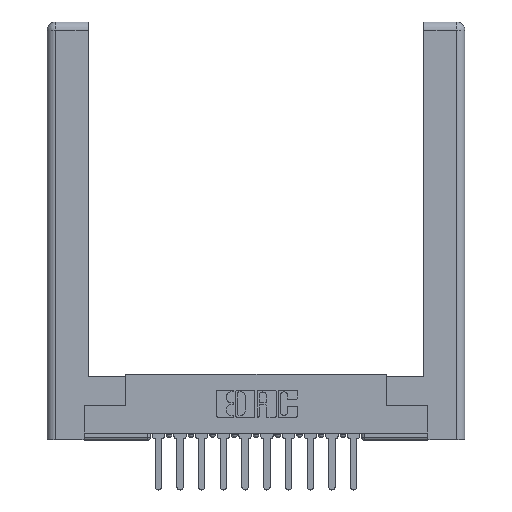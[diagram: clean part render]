
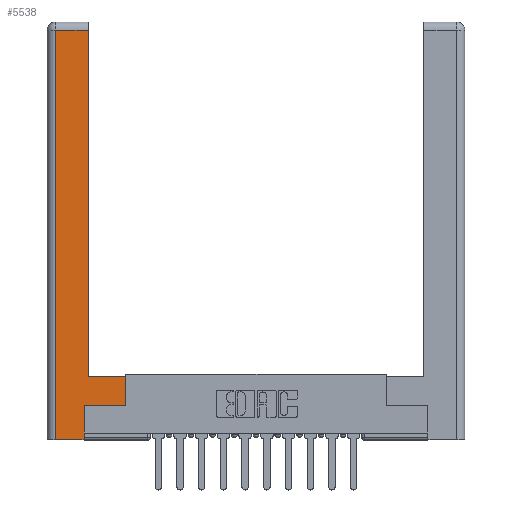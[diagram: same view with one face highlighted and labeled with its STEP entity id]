
A CAD part, top view. The second image highlights one B-rep face of the part: STEP entity #5538.
In plain terms, the highlighted planar face has unit normal (0, 0, 1).
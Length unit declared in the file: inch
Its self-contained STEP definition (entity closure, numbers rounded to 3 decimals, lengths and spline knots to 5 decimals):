
#361 = ORIENTED_EDGE ( 'NONE', *, *, #8098, .T. ) ;
#816 = VECTOR ( 'NONE', #12242, 39.37008 ) ;
#1055 = EDGE_CURVE ( 'NONE', #7611, #7366, #11039, .T. ) ;
#1480 = CARTESIAN_POINT ( 'NONE',  ( 0., 0., 0. ) ) ;
#1547 = CARTESIAN_POINT ( 'NONE',  ( 0.265, 0., 0. ) ) ;
#1591 = CARTESIAN_POINT ( 'NONE',  ( 0.0615, 0., 0. ) ) ;
#1677 = DIRECTION ( 'NONE',  ( 0., 1., 0. ) ) ;
#1828 = CARTESIAN_POINT ( 'NONE',  ( 0.0615, 2.94, 0. ) ) ;
#2106 = CARTESIAN_POINT ( 'NONE',  ( 0.565, 0.45, 0. ) ) ;
#3268 = CARTESIAN_POINT ( 'NONE',  ( 0.265, 0., 0. ) ) ;
#3438 = CARTESIAN_POINT ( 'NONE',  ( 0.295, 2.94, 0. ) ) ;
#3465 = VERTEX_POINT ( 'NONE', #11208 ) ;
#3565 = EDGE_CURVE ( 'NONE', #9347, #11567, #4150, .T. ) ;
#4096 = CARTESIAN_POINT ( 'NONE',  ( 0.295, 3., 0. ) ) ;
#4128 = DIRECTION ( 'NONE',  ( 0., 1., 0. ) ) ;
#4150 = LINE ( 'NONE', #1591, #12710 ) ;
#4810 = EDGE_CURVE ( 'NONE', #3465, #8582, #5260, .T. ) ;
#4844 = VECTOR ( 'NONE', #13794, 39.37008 ) ;
#4939 = CARTESIAN_POINT ( 'NONE',  ( 0.565, 0.245, 0. ) ) ;
#4995 = LINE ( 'NONE', #14581, #12330 ) ;
#5260 = LINE ( 'NONE', #4096, #816 ) ;
#5538 = ADVANCED_FACE ( 'NONE', ( #8368 ), #12187, .F. ) ;
#5605 = ORIENTED_EDGE ( 'NONE', *, *, #9358, .T. ) ;
#5918 = CARTESIAN_POINT ( 'NONE',  ( 0.265, 0.245, 0. ) ) ;
#5971 = VERTEX_POINT ( 'NONE', #3268 ) ;
#6779 = VECTOR ( 'NONE', #10830, 39.37008 ) ;
#7082 = LINE ( 'NONE', #4939, #6779 ) ;
#7221 = VERTEX_POINT ( 'NONE', #5918 ) ;
#7317 = EDGE_LOOP ( 'NONE', ( #14243, #361, #14597, #12318, #5605, #9285, #11710, #10459 ) ) ;
#7365 = VECTOR ( 'NONE', #4128, 39.37008 ) ;
#7366 = VERTEX_POINT ( 'NONE', #2106 ) ;
#7581 = CARTESIAN_POINT ( 'NONE',  ( 0.565, 0.45, 0. ) ) ;
#7611 = VERTEX_POINT ( 'NONE', #9022 ) ;
#7762 = LINE ( 'NONE', #1828, #4844 ) ;
#8098 = EDGE_CURVE ( 'NONE', #8582, #9347, #7762, .T. ) ;
#8368 = FACE_OUTER_BOUND ( 'NONE', #7317, .T. ) ;
#8582 = VERTEX_POINT ( 'NONE', #3438 ) ;
#8612 = DIRECTION ( 'NONE',  ( -1., 0., 0. ) ) ;
#8720 = VECTOR ( 'NONE', #1677, 39.37008 ) ;
#8926 = DIRECTION ( 'NONE',  ( 0., -1., 0. ) ) ;
#9022 = CARTESIAN_POINT ( 'NONE',  ( 0.565, 0.245, 0. ) ) ;
#9263 = VECTOR ( 'NONE', #13666, 39.37008 ) ;
#9285 = ORIENTED_EDGE ( 'NONE', *, *, #12001, .T. ) ;
#9347 = VERTEX_POINT ( 'NONE', #10344 ) ;
#9358 = EDGE_CURVE ( 'NONE', #5971, #7221, #14982, .T. ) ;
#10344 = CARTESIAN_POINT ( 'NONE',  ( 0.0615, 2.94, 0. ) ) ;
#10459 = ORIENTED_EDGE ( 'NONE', *, *, #13831, .T. ) ;
#10830 = DIRECTION ( 'NONE',  ( 1., 0., 0. ) ) ;
#10952 = AXIS2_PLACEMENT_3D ( 'NONE', #1480, #13151, #10951 ) ;
#10951 = DIRECTION ( 'NONE',  ( -1., 0., 0. ) ) ;
#11039 = LINE ( 'NONE', #7581, #7365 ) ;
#11208 = CARTESIAN_POINT ( 'NONE',  ( 0.295, 0.45, 0. ) ) ;
#11298 = EDGE_CURVE ( 'NONE', #11567, #5971, #14931, .T. ) ;
#11454 = CARTESIAN_POINT ( 'NONE',  ( 0.265, 0.245, 0. ) ) ;
#11567 = VERTEX_POINT ( 'NONE', #15402 ) ;
#11710 = ORIENTED_EDGE ( 'NONE', *, *, #1055, .T. ) ;
#12001 = EDGE_CURVE ( 'NONE', #7221, #7611, #7082, .T. ) ;
#12187 = PLANE ( 'NONE',  #10952 ) ;
#12242 = DIRECTION ( 'NONE',  ( 0., 1., 0. ) ) ;
#12318 = ORIENTED_EDGE ( 'NONE', *, *, #11298, .T. ) ;
#12330 = VECTOR ( 'NONE', #8612, 39.37008 ) ;
#12710 = VECTOR ( 'NONE', #8926, 39.37008 ) ;
#13151 = DIRECTION ( 'NONE',  ( 0., 0., -1. ) ) ;
#13666 = DIRECTION ( 'NONE',  ( 1., 0., 0. ) ) ;
#13794 = DIRECTION ( 'NONE',  ( -1., 0., 0. ) ) ;
#13831 = EDGE_CURVE ( 'NONE', #7366, #3465, #4995, .T. ) ;
#14243 = ORIENTED_EDGE ( 'NONE', *, *, #4810, .T. ) ;
#14581 = CARTESIAN_POINT ( 'NONE',  ( 0.295, 0.45, 0. ) ) ;
#14597 = ORIENTED_EDGE ( 'NONE', *, *, #3565, .T. ) ;
#14931 = LINE ( 'NONE', #1547, #9263 ) ;
#14982 = LINE ( 'NONE', #11454, #8720 ) ;
#15402 = CARTESIAN_POINT ( 'NONE',  ( 0.0615, 0., 0. ) ) ;
